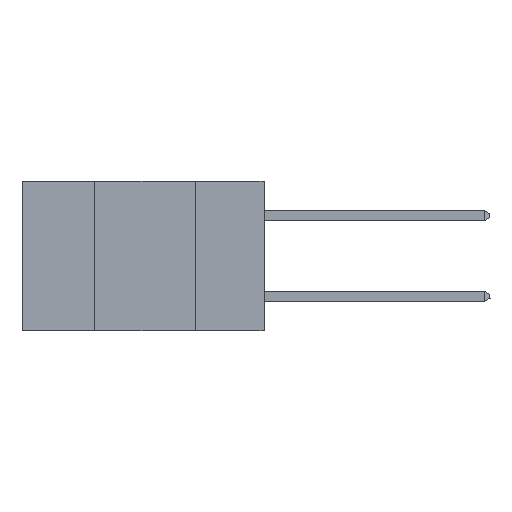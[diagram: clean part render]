
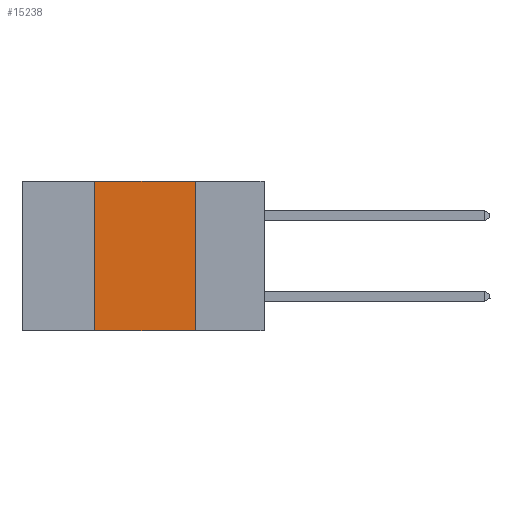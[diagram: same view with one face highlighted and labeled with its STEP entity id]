
A CAD part, left-side view. The second image highlights one B-rep face of the part: STEP entity #15238.
In plain terms, the highlighted planar face has unit normal (-1, 0, 0).
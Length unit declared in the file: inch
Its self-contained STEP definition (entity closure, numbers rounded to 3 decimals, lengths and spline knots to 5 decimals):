
#548 = DIRECTION ( 'NONE',  ( 0., -1., 0. ) ) ;
#857 = VERTEX_POINT ( 'NONE', #18036 ) ;
#1140 = DIRECTION ( 'NONE',  ( 0., 0., -1. ) ) ;
#3375 = CARTESIAN_POINT ( 'NONE',  ( 0., 0.17, 0. ) ) ;
#3507 = PLANE ( 'NONE',  #30072 ) ;
#3998 = EDGE_CURVE ( 'NONE', #27463, #28681, #29574, .T. ) ;
#4374 = ORIENTED_EDGE ( 'NONE', *, *, #3998, .F. ) ;
#5029 = EDGE_CURVE ( 'NONE', #857, #15153, #26394, .T. ) ;
#5150 = ORIENTED_EDGE ( 'NONE', *, *, #20187, .F. ) ;
#5395 = CARTESIAN_POINT ( 'NONE',  ( 0., 0.42, 0. ) ) ;
#5547 = CARTESIAN_POINT ( 'NONE',  ( 0., 0.17, 0. ) ) ;
#5888 = DIRECTION ( 'NONE',  ( 0., 0., -1. ) ) ;
#6568 = CARTESIAN_POINT ( 'NONE',  ( 0., 0.42, 0. ) ) ;
#8476 = CARTESIAN_POINT ( 'NONE',  ( 0., 0.6, 0. ) ) ;
#10414 = EDGE_LOOP ( 'NONE', ( #5150, #4374, #13296, #12516 ) ) ;
#11002 = CARTESIAN_POINT ( 'NONE',  ( 0., 0.6, 0. ) ) ;
#12439 = EDGE_CURVE ( 'NONE', #857, #27463, #29732, .T. ) ;
#12516 = ORIENTED_EDGE ( 'NONE', *, *, #5029, .T. ) ;
#13041 = CARTESIAN_POINT ( 'NONE',  ( 0., 0.6, -0.37 ) ) ;
#13296 = ORIENTED_EDGE ( 'NONE', *, *, #12439, .F. ) ;
#15153 = VERTEX_POINT ( 'NONE', #18151 ) ;
#15238 = ADVANCED_FACE ( 'NONE', ( #18872 ), #3507, .F. ) ;
#15979 = DIRECTION ( 'NONE',  ( 1., 0., 0. ) ) ;
#16515 = VECTOR ( 'NONE', #20233, 39.37008 ) ;
#17122 = VECTOR ( 'NONE', #25663, 39.37008 ) ;
#18036 = CARTESIAN_POINT ( 'NONE',  ( 0., 0.42, -0.37 ) ) ;
#18151 = CARTESIAN_POINT ( 'NONE',  ( 0., 0.17, -0.37 ) ) ;
#18872 = FACE_OUTER_BOUND ( 'NONE', #10414, .T. ) ;
#20187 = EDGE_CURVE ( 'NONE', #28681, #15153, #23165, .T. ) ;
#20233 = DIRECTION ( 'NONE',  ( 0., 0., 1. ) ) ;
#22386 = VECTOR ( 'NONE', #5888, 39.37008 ) ;
#23165 = LINE ( 'NONE', #3375, #22386 ) ;
#25635 = VECTOR ( 'NONE', #548, 39.37008 ) ;
#25663 = DIRECTION ( 'NONE',  ( 0., -1., 0. ) ) ;
#26394 = LINE ( 'NONE', #13041, #25635 ) ;
#27463 = VERTEX_POINT ( 'NONE', #6568 ) ;
#28681 = VERTEX_POINT ( 'NONE', #5547 ) ;
#29574 = LINE ( 'NONE', #8476, #17122 ) ;
#29732 = LINE ( 'NONE', #5395, #16515 ) ;
#30072 = AXIS2_PLACEMENT_3D ( 'NONE', #11002, #15979, #1140 ) ;
